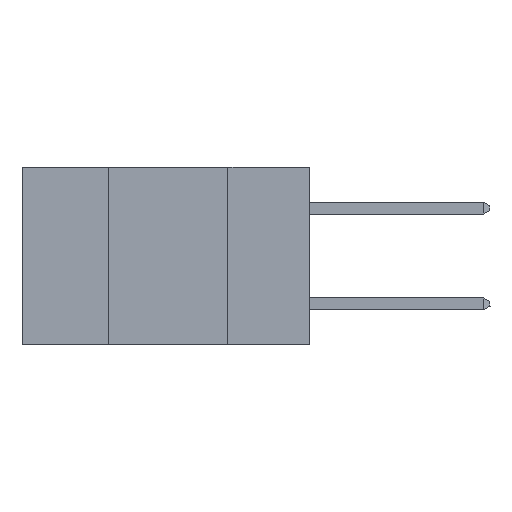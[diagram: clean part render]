
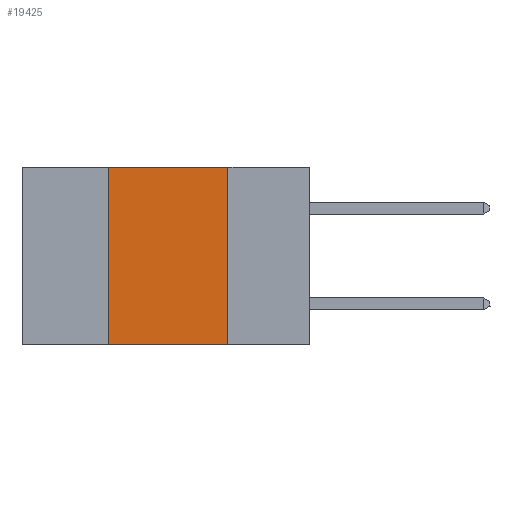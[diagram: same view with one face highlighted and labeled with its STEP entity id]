
A CAD part, left-side view. The second image highlights one B-rep face of the part: STEP entity #19425.
In plain terms, the highlighted planar face has unit normal (-1, 0, 0).
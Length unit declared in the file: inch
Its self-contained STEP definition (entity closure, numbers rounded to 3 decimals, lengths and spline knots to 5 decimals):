
#264 = CARTESIAN_POINT ( 'NONE',  ( 0., 0.6, 0. ) ) ;
#526 = FACE_OUTER_BOUND ( 'NONE', #13482, .T. ) ;
#1101 = ORIENTED_EDGE ( 'NONE', *, *, #1573, .T. ) ;
#1573 = EDGE_CURVE ( 'NONE', #18251, #9691, #10099, .T. ) ;
#3205 = CARTESIAN_POINT ( 'NONE',  ( 0., 0.6, -0.37 ) ) ;
#3341 = LINE ( 'NONE', #9277, #20375 ) ;
#3884 = EDGE_CURVE ( 'NONE', #9365, #9691, #3341, .T. ) ;
#4122 = EDGE_CURVE ( 'NONE', #18251, #10835, #20641, .T. ) ;
#4544 = AXIS2_PLACEMENT_3D ( 'NONE', #16873, #4716, #9770 ) ;
#4716 = DIRECTION ( 'NONE',  ( 1., 0., 0. ) ) ;
#6335 = VECTOR ( 'NONE', #13410, 39.37008 ) ;
#7936 = PLANE ( 'NONE',  #4544 ) ;
#8059 = VECTOR ( 'NONE', #14343, 39.37008 ) ;
#9277 = CARTESIAN_POINT ( 'NONE',  ( 0., 0.17, 0. ) ) ;
#9365 = VERTEX_POINT ( 'NONE', #12421 ) ;
#9691 = VERTEX_POINT ( 'NONE', #21866 ) ;
#9770 = DIRECTION ( 'NONE',  ( 0., 0., -1. ) ) ;
#9960 = DIRECTION ( 'NONE',  ( 0., -1., 0. ) ) ;
#10099 = LINE ( 'NONE', #3205, #17296 ) ;
#10835 = VERTEX_POINT ( 'NONE', #18385 ) ;
#11557 = EDGE_CURVE ( 'NONE', #10835, #9365, #12177, .T. ) ;
#12177 = LINE ( 'NONE', #264, #8059 ) ;
#12421 = CARTESIAN_POINT ( 'NONE',  ( 0., 0.17, 0. ) ) ;
#13410 = DIRECTION ( 'NONE',  ( 0., 0., 1. ) ) ;
#13482 = EDGE_LOOP ( 'NONE', ( #14129, #18163, #18295, #1101 ) ) ;
#14129 = ORIENTED_EDGE ( 'NONE', *, *, #3884, .F. ) ;
#14332 = CARTESIAN_POINT ( 'NONE',  ( 0., 0.42, 0. ) ) ;
#14343 = DIRECTION ( 'NONE',  ( 0., -1., 0. ) ) ;
#16873 = CARTESIAN_POINT ( 'NONE',  ( 0., 0.6, 0. ) ) ;
#17296 = VECTOR ( 'NONE', #9960, 39.37008 ) ;
#18163 = ORIENTED_EDGE ( 'NONE', *, *, #11557, .F. ) ;
#18251 = VERTEX_POINT ( 'NONE', #21913 ) ;
#18295 = ORIENTED_EDGE ( 'NONE', *, *, #4122, .F. ) ;
#18385 = CARTESIAN_POINT ( 'NONE',  ( 0., 0.42, 0. ) ) ;
#19425 = ADVANCED_FACE ( 'NONE', ( #526 ), #7936, .F. ) ;
#20375 = VECTOR ( 'NONE', #21555, 39.37008 ) ;
#20641 = LINE ( 'NONE', #14332, #6335 ) ;
#21555 = DIRECTION ( 'NONE',  ( 0., 0., -1. ) ) ;
#21866 = CARTESIAN_POINT ( 'NONE',  ( 0., 0.17, -0.37 ) ) ;
#21913 = CARTESIAN_POINT ( 'NONE',  ( 0., 0.42, -0.37 ) ) ;
